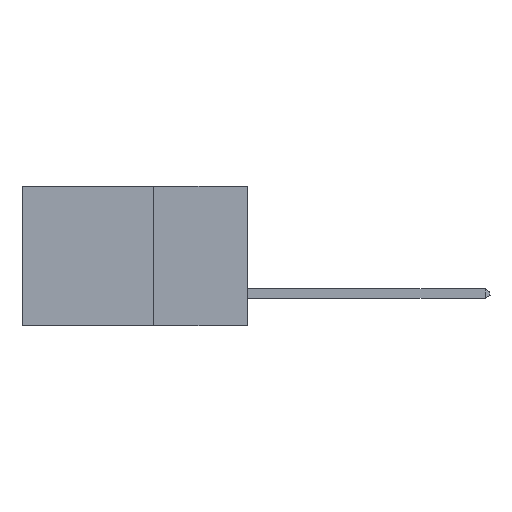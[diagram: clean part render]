
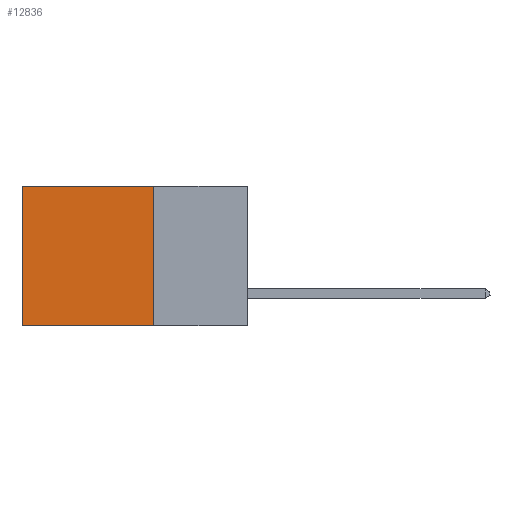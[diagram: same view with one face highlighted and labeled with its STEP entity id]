
A CAD part, left-side view. The second image highlights one B-rep face of the part: STEP entity #12836.
In plain terms, the highlighted planar face has unit normal (-1, 0, 0).
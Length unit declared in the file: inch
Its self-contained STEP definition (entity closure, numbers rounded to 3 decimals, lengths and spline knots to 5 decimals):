
#111 = CARTESIAN_POINT ( 'NONE',  ( 0.298, 0.25, -0.37 ) ) ;
#223 = ORIENTED_EDGE ( 'NONE', *, *, #24933, .T. ) ;
#490 = DIRECTION ( 'NONE',  ( 1., 0., 0. ) ) ;
#558 = CARTESIAN_POINT ( 'NONE',  ( 0.298, 0.25, -0.37 ) ) ;
#824 = CARTESIAN_POINT ( 'NONE',  ( 0.298, 0.6, -0.37 ) ) ;
#2933 = CARTESIAN_POINT ( 'NONE',  ( 0.298, 0.25, 0. ) ) ;
#3661 = EDGE_CURVE ( 'NONE', #23434, #16337, #14125, .T. ) ;
#4215 = CARTESIAN_POINT ( 'NONE',  ( 0.298, 0.25, 0. ) ) ;
#4408 = VECTOR ( 'NONE', #11551, 39.37008 ) ;
#5069 = ORIENTED_EDGE ( 'NONE', *, *, #13033, .F. ) ;
#8148 = DIRECTION ( 'NONE',  ( 0., 1., 0. ) ) ;
#8357 = VERTEX_POINT ( 'NONE', #16916 ) ;
#11551 = DIRECTION ( 'NONE',  ( 0., 0., -1. ) ) ;
#12774 = CARTESIAN_POINT ( 'NONE',  ( 0.298, 0.25, 0. ) ) ;
#12836 = ADVANCED_FACE ( 'NONE', ( #14077 ), #27687, .F. ) ;
#13033 = EDGE_CURVE ( 'NONE', #17971, #23434, #25986, .T. ) ;
#13460 = CARTESIAN_POINT ( 'NONE',  ( 0.298, 0.25, 0. ) ) ;
#14077 = FACE_OUTER_BOUND ( 'NONE', #14121, .T. ) ;
#14121 = EDGE_LOOP ( 'NONE', ( #19471, #21244, #5069, #223 ) ) ;
#14125 = LINE ( 'NONE', #558, #27596 ) ;
#15501 = VECTOR ( 'NONE', #15665, 39.37008 ) ;
#15524 = DIRECTION ( 'NONE',  ( 0., 0., -1. ) ) ;
#15665 = DIRECTION ( 'NONE',  ( 0., 0., -1. ) ) ;
#16337 = VERTEX_POINT ( 'NONE', #824 ) ;
#16916 = CARTESIAN_POINT ( 'NONE',  ( 0.298, 0.6, 0. ) ) ;
#17971 = VERTEX_POINT ( 'NONE', #13460 ) ;
#19378 = LINE ( 'NONE', #30386, #15501 ) ;
#19471 = ORIENTED_EDGE ( 'NONE', *, *, #30853, .T. ) ;
#20208 = LINE ( 'NONE', #2933, #26742 ) ;
#21244 = ORIENTED_EDGE ( 'NONE', *, *, #3661, .F. ) ;
#23434 = VERTEX_POINT ( 'NONE', #111 ) ;
#24933 = EDGE_CURVE ( 'NONE', #17971, #8357, #20208, .T. ) ;
#25986 = LINE ( 'NONE', #4215, #4408 ) ;
#26429 = DIRECTION ( 'NONE',  ( 0., 1., 0. ) ) ;
#26742 = VECTOR ( 'NONE', #26429, 39.37008 ) ;
#27596 = VECTOR ( 'NONE', #8148, 39.37008 ) ;
#27687 = PLANE ( 'NONE',  #31470 ) ;
#30386 = CARTESIAN_POINT ( 'NONE',  ( 0.298, 0.6, 0. ) ) ;
#30853 = EDGE_CURVE ( 'NONE', #8357, #16337, #19378, .T. ) ;
#31470 = AXIS2_PLACEMENT_3D ( 'NONE', #12774, #490, #15524 ) ;
